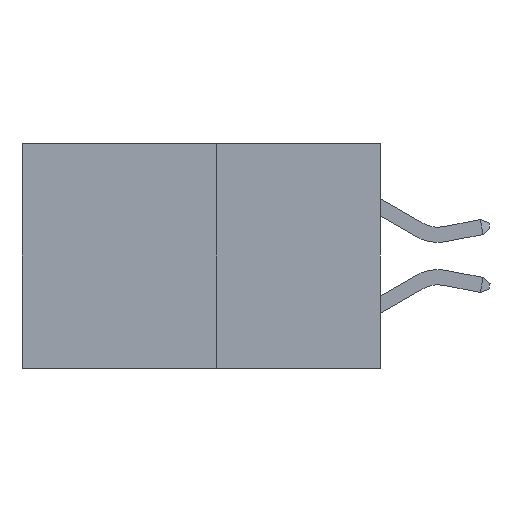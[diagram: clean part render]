
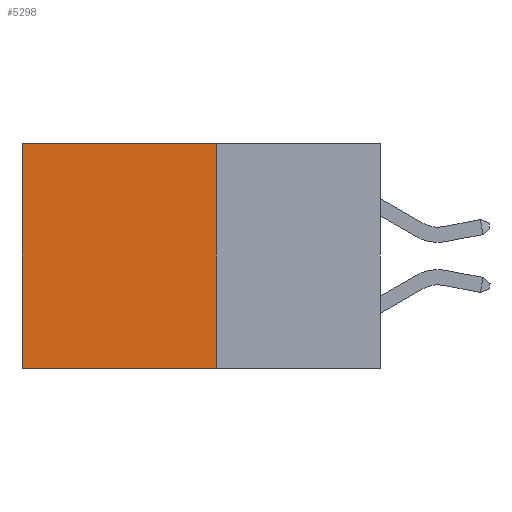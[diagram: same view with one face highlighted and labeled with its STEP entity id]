
A CAD part, left-side view. The second image highlights one B-rep face of the part: STEP entity #5298.
In plain terms, the highlighted planar face has unit normal (-1, 0, 0).
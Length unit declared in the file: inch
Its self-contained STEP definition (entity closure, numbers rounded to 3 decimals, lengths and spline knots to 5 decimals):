
#908 = VECTOR ( 'NONE', #12397, 39.37008 ) ;
#1178 = ORIENTED_EDGE ( 'NONE', *, *, #14448, .F. ) ;
#2045 = LINE ( 'NONE', #3804, #8764 ) ;
#2470 = ORIENTED_EDGE ( 'NONE', *, *, #10219, .T. ) ;
#2867 = DIRECTION ( 'NONE',  ( 0., 0., -1. ) ) ;
#2958 = AXIS2_PLACEMENT_3D ( 'NONE', #8587, #13624, #6753 ) ;
#3001 = CARTESIAN_POINT ( 'NONE',  ( 0.277, 0.59, -0.37 ) ) ;
#3735 = CARTESIAN_POINT ( 'NONE',  ( 0.277, 0.27, -0.37 ) ) ;
#3804 = CARTESIAN_POINT ( 'NONE',  ( 0.277, 0.27, 0. ) ) ;
#4367 = LINE ( 'NONE', #7079, #11103 ) ;
#4634 = EDGE_CURVE ( 'NONE', #16380, #15721, #8841, .T. ) ;
#5243 = VERTEX_POINT ( 'NONE', #11022 ) ;
#5298 = ADVANCED_FACE ( 'NONE', ( #5878 ), #8516, .F. ) ;
#5741 = DIRECTION ( 'NONE',  ( 0., 1., 0. ) ) ;
#5878 = FACE_OUTER_BOUND ( 'NONE', #12081, .T. ) ;
#6753 = DIRECTION ( 'NONE',  ( 0., 0., -1. ) ) ;
#7079 = CARTESIAN_POINT ( 'NONE',  ( 0.277, 0.27, -0.37 ) ) ;
#8502 = CARTESIAN_POINT ( 'NONE',  ( 0.277, 0.59, -0.37 ) ) ;
#8516 = PLANE ( 'NONE',  #2958 ) ;
#8587 = CARTESIAN_POINT ( 'NONE',  ( 0.277, 0.27, -0.37 ) ) ;
#8764 = VECTOR ( 'NONE', #11855, 39.37008 ) ;
#8841 = LINE ( 'NONE', #3735, #15559 ) ;
#9524 = ORIENTED_EDGE ( 'NONE', *, *, #12277, .T. ) ;
#10219 = EDGE_CURVE ( 'NONE', #16380, #5243, #2045, .T. ) ;
#10351 = CARTESIAN_POINT ( 'NONE',  ( 0.277, 0.27, -0.37 ) ) ;
#11022 = CARTESIAN_POINT ( 'NONE',  ( 0.277, 0.59, 0. ) ) ;
#11103 = VECTOR ( 'NONE', #5741, 39.37008 ) ;
#11208 = LINE ( 'NONE', #3001, #908 ) ;
#11855 = DIRECTION ( 'NONE',  ( 0., 1., 0. ) ) ;
#12031 = ORIENTED_EDGE ( 'NONE', *, *, #4634, .F. ) ;
#12081 = EDGE_LOOP ( 'NONE', ( #9524, #1178, #12031, #2470 ) ) ;
#12277 = EDGE_CURVE ( 'NONE', #5243, #16148, #11208, .T. ) ;
#12397 = DIRECTION ( 'NONE',  ( 0., 0., -1. ) ) ;
#12968 = CARTESIAN_POINT ( 'NONE',  ( 0.277, 0.27, 0. ) ) ;
#13624 = DIRECTION ( 'NONE',  ( 1., 0., 0. ) ) ;
#14448 = EDGE_CURVE ( 'NONE', #15721, #16148, #4367, .T. ) ;
#15559 = VECTOR ( 'NONE', #2867, 39.37008 ) ;
#15721 = VERTEX_POINT ( 'NONE', #10351 ) ;
#16148 = VERTEX_POINT ( 'NONE', #8502 ) ;
#16380 = VERTEX_POINT ( 'NONE', #12968 ) ;
